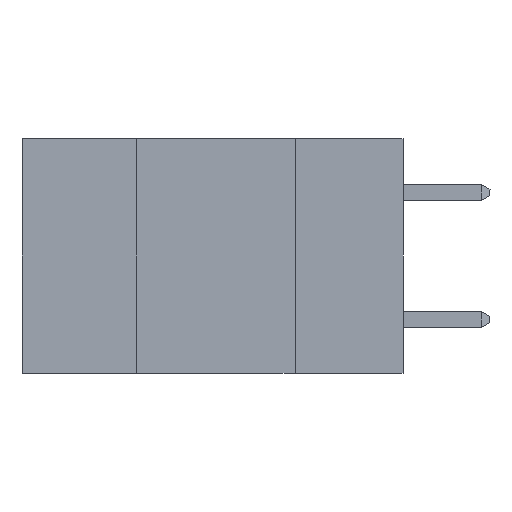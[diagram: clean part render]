
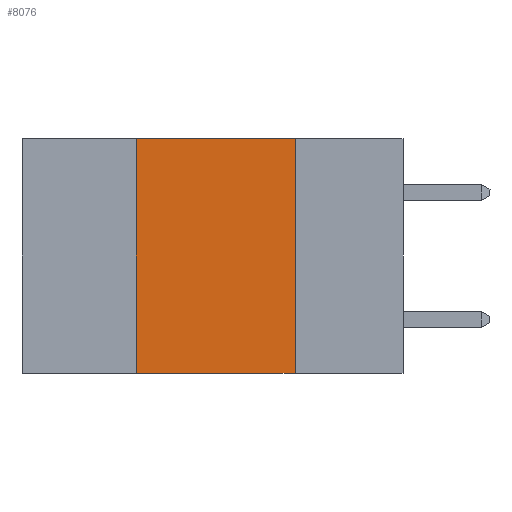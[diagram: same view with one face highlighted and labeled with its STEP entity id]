
A CAD part, left-side view. The second image highlights one B-rep face of the part: STEP entity #8076.
In plain terms, the highlighted planar face has unit normal (-1, 0, 0).
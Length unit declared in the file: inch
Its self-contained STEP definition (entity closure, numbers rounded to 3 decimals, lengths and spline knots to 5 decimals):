
#298 = LINE ( 'NONE', #8427, #1927 ) ;
#473 = VERTEX_POINT ( 'NONE', #6560 ) ;
#793 = CARTESIAN_POINT ( 'NONE',  ( 0., 0.6, 0. ) ) ;
#966 = VERTEX_POINT ( 'NONE', #4849 ) ;
#1183 = ORIENTED_EDGE ( 'NONE', *, *, #2490, .F. ) ;
#1510 = DIRECTION ( 'NONE',  ( 1., 0., 0. ) ) ;
#1537 = VERTEX_POINT ( 'NONE', #5348 ) ;
#1554 = LINE ( 'NONE', #7612, #1878 ) ;
#1685 = EDGE_CURVE ( 'NONE', #966, #6678, #1554, .T. ) ;
#1776 = DIRECTION ( 'NONE',  ( 0., 0., -1. ) ) ;
#1878 = VECTOR ( 'NONE', #8419, 39.37008 ) ;
#1927 = VECTOR ( 'NONE', #6224, 39.37008 ) ;
#2426 = ORIENTED_EDGE ( 'NONE', *, *, #1685, .F. ) ;
#2490 = EDGE_CURVE ( 'NONE', #1537, #966, #6350, .T. ) ;
#2861 = VECTOR ( 'NONE', #1776, 39.37008 ) ;
#3015 = EDGE_LOOP ( 'NONE', ( #8091, #2426, #1183, #6622 ) ) ;
#3114 = CARTESIAN_POINT ( 'NONE',  ( 0., 0.17, 0. ) ) ;
#3493 = CARTESIAN_POINT ( 'NONE',  ( 0., 0.42, 0. ) ) ;
#3816 = DIRECTION ( 'NONE',  ( 0., 0., -1. ) ) ;
#4170 = EDGE_CURVE ( 'NONE', #1537, #473, #298, .T. ) ;
#4215 = DIRECTION ( 'NONE',  ( 0., 0., 1. ) ) ;
#4849 = CARTESIAN_POINT ( 'NONE',  ( 0., 0.42, 0. ) ) ;
#5348 = CARTESIAN_POINT ( 'NONE',  ( 0., 0.42, -0.37 ) ) ;
#6224 = DIRECTION ( 'NONE',  ( 0., -1., 0. ) ) ;
#6341 = EDGE_CURVE ( 'NONE', #6678, #473, #8151, .T. ) ;
#6350 = LINE ( 'NONE', #3493, #7399 ) ;
#6360 = FACE_OUTER_BOUND ( 'NONE', #3015, .T. ) ;
#6377 = AXIS2_PLACEMENT_3D ( 'NONE', #793, #1510, #3816 ) ;
#6560 = CARTESIAN_POINT ( 'NONE',  ( 0., 0.17, -0.37 ) ) ;
#6622 = ORIENTED_EDGE ( 'NONE', *, *, #4170, .T. ) ;
#6678 = VERTEX_POINT ( 'NONE', #7587 ) ;
#7399 = VECTOR ( 'NONE', #4215, 39.37008 ) ;
#7587 = CARTESIAN_POINT ( 'NONE',  ( 0., 0.17, 0. ) ) ;
#7612 = CARTESIAN_POINT ( 'NONE',  ( 0., 0.6, 0. ) ) ;
#8076 = ADVANCED_FACE ( 'NONE', ( #6360 ), #8486, .F. ) ;
#8091 = ORIENTED_EDGE ( 'NONE', *, *, #6341, .F. ) ;
#8151 = LINE ( 'NONE', #3114, #2861 ) ;
#8419 = DIRECTION ( 'NONE',  ( 0., -1., 0. ) ) ;
#8427 = CARTESIAN_POINT ( 'NONE',  ( 0., 0.6, -0.37 ) ) ;
#8486 = PLANE ( 'NONE',  #6377 ) ;
